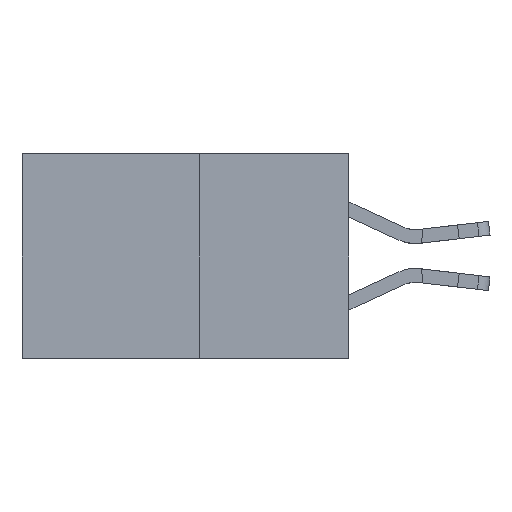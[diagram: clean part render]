
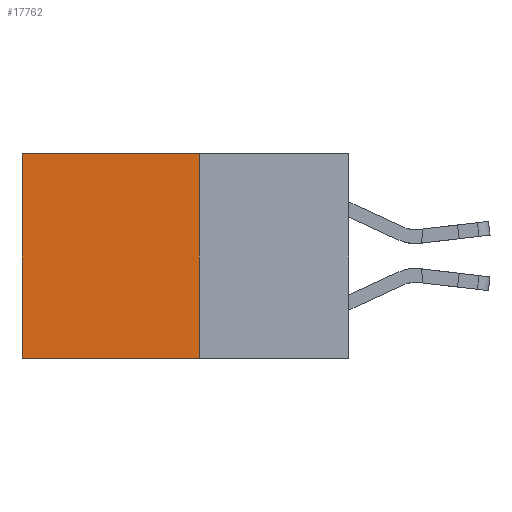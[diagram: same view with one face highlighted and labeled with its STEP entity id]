
A CAD part, left-side view. The second image highlights one B-rep face of the part: STEP entity #17762.
In plain terms, the highlighted planar face has unit normal (-1, 0, 0).
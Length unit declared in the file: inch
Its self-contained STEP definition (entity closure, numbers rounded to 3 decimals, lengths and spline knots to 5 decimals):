
#1072 = LINE ( 'NONE', #3690, #6478 ) ;
#1822 = ORIENTED_EDGE ( 'NONE', *, *, #29140, .F. ) ;
#3690 = CARTESIAN_POINT ( 'NONE',  ( 0.277, 0.27, 0. ) ) ;
#4174 = ORIENTED_EDGE ( 'NONE', *, *, #13921, .T. ) ;
#4903 = VERTEX_POINT ( 'NONE', #16376 ) ;
#5396 = CARTESIAN_POINT ( 'NONE',  ( 0.277, 0.27, 0. ) ) ;
#6478 = VECTOR ( 'NONE', #15278, 39.37008 ) ;
#7010 = CARTESIAN_POINT ( 'NONE',  ( 0.277, 0.27, -0.37 ) ) ;
#8289 = VECTOR ( 'NONE', #25581, 39.37008 ) ;
#8329 = VERTEX_POINT ( 'NONE', #5396 ) ;
#9270 = VERTEX_POINT ( 'NONE', #10915 ) ;
#9652 = CARTESIAN_POINT ( 'NONE',  ( 0.277, 0.59, -0.37 ) ) ;
#10044 = PLANE ( 'NONE',  #26614 ) ;
#10915 = CARTESIAN_POINT ( 'NONE',  ( 0.277, 0.27, -0.37 ) ) ;
#12396 = DIRECTION ( 'NONE',  ( 1., 0., 0. ) ) ;
#12845 = VERTEX_POINT ( 'NONE', #18836 ) ;
#13395 = VECTOR ( 'NONE', #25782, 39.37008 ) ;
#13921 = EDGE_CURVE ( 'NONE', #8329, #4903, #1072, .T. ) ;
#14842 = FACE_OUTER_BOUND ( 'NONE', #19904, .T. ) ;
#15278 = DIRECTION ( 'NONE',  ( 0., 1., 0. ) ) ;
#16373 = CARTESIAN_POINT ( 'NONE',  ( 0.277, 0.27, -0.37 ) ) ;
#16376 = CARTESIAN_POINT ( 'NONE',  ( 0.277, 0.59, 0. ) ) ;
#17553 = EDGE_CURVE ( 'NONE', #9270, #12845, #26067, .T. ) ;
#17645 = EDGE_CURVE ( 'NONE', #4903, #12845, #23894, .T. ) ;
#17762 = ADVANCED_FACE ( 'NONE', ( #14842 ), #10044, .F. ) ;
#17940 = VECTOR ( 'NONE', #23351, 39.37008 ) ;
#18836 = CARTESIAN_POINT ( 'NONE',  ( 0.277, 0.59, -0.37 ) ) ;
#19904 = EDGE_LOOP ( 'NONE', ( #19948, #23335, #1822, #4174 ) ) ;
#19948 = ORIENTED_EDGE ( 'NONE', *, *, #17645, .T. ) ;
#23335 = ORIENTED_EDGE ( 'NONE', *, *, #17553, .F. ) ;
#23351 = DIRECTION ( 'NONE',  ( 0., 0., -1. ) ) ;
#23894 = LINE ( 'NONE', #9652, #13395 ) ;
#25581 = DIRECTION ( 'NONE',  ( 0., 1., 0. ) ) ;
#25782 = DIRECTION ( 'NONE',  ( 0., 0., -1. ) ) ;
#26067 = LINE ( 'NONE', #7010, #8289 ) ;
#26283 = CARTESIAN_POINT ( 'NONE',  ( 0.277, 0.27, -0.37 ) ) ;
#26614 = AXIS2_PLACEMENT_3D ( 'NONE', #26283, #12396, #28592 ) ;
#28592 = DIRECTION ( 'NONE',  ( 0., 0., -1. ) ) ;
#29140 = EDGE_CURVE ( 'NONE', #8329, #9270, #29506, .T. ) ;
#29506 = LINE ( 'NONE', #16373, #17940 ) ;
